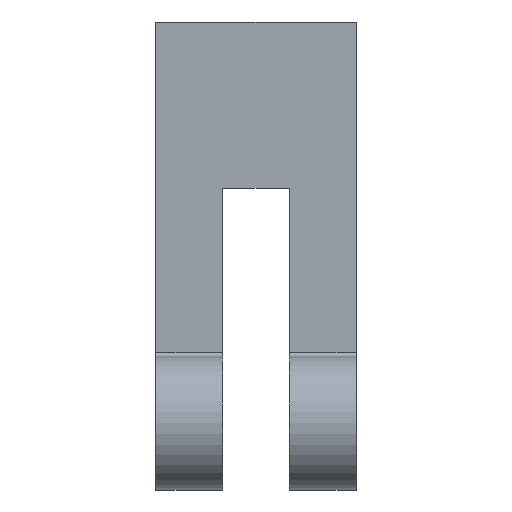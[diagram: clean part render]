
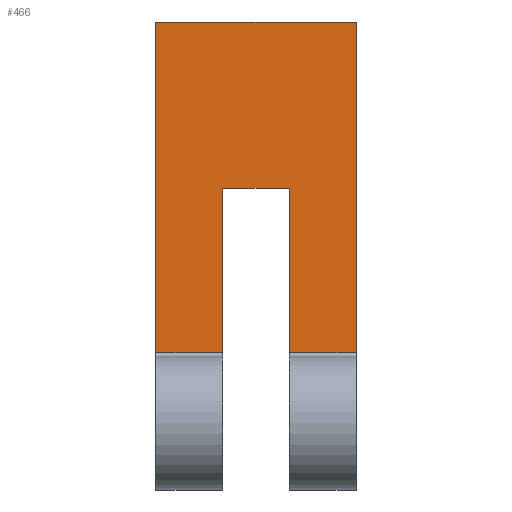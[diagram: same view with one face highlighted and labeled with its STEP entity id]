
A CAD part, top view. The second image highlights one B-rep face of the part: STEP entity #466.
In plain terms, the highlighted planar face has unit normal (0, 0, 1).
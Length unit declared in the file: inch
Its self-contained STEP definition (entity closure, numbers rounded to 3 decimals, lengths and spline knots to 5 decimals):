
#29=PLANE('',#520);
#52=FACE_OUTER_BOUND('',#76,.T.);
#76=EDGE_LOOP('',(#421,#422,#423,#424,#425,#426,#427,#428));
#80=LINE('',#664,#130);
#81=LINE('',#670,#131);
#91=LINE('',#705,#141);
#103=LINE('',#731,#153);
#124=LINE('',#778,#174);
#125=LINE('',#781,#175);
#127=LINE('',#784,#177);
#128=LINE('',#787,#178);
#130=VECTOR('',#532,0.3937);
#131=VECTOR('',#537,0.3937);
#141=VECTOR('',#567,0.3937);
#153=VECTOR('',#587,0.3937);
#174=VECTOR('',#638,0.3937);
#175=VECTOR('',#641,0.3937);
#177=VECTOR('',#645,0.3937);
#178=VECTOR('',#650,0.3937);
#195=VERTEX_POINT('',#657);
#198=VERTEX_POINT('',#662);
#200=VERTEX_POINT('',#667);
#201=VERTEX_POINT('',#669);
#216=VERTEX_POINT('',#704);
#226=VERTEX_POINT('',#730);
#237=VERTEX_POINT('',#776);
#238=VERTEX_POINT('',#780);
#242=EDGE_CURVE('',#195,#198,#80,.T.);
#244=EDGE_CURVE('',#201,#200,#81,.T.);
#261=EDGE_CURVE('',#216,#195,#91,.T.);
#275=EDGE_CURVE('',#201,#226,#103,.T.);
#299=EDGE_CURVE('',#237,#198,#124,.T.);
#300=EDGE_CURVE('',#238,#216,#125,.T.);
#302=EDGE_CURVE('',#200,#238,#127,.T.);
#304=EDGE_CURVE('',#226,#237,#128,.T.);
#421=ORIENTED_EDGE('',*,*,#242,.T.);
#422=ORIENTED_EDGE('',*,*,#299,.F.);
#423=ORIENTED_EDGE('',*,*,#304,.F.);
#424=ORIENTED_EDGE('',*,*,#275,.F.);
#425=ORIENTED_EDGE('',*,*,#244,.T.);
#426=ORIENTED_EDGE('',*,*,#302,.T.);
#427=ORIENTED_EDGE('',*,*,#300,.T.);
#428=ORIENTED_EDGE('',*,*,#261,.T.);
#466=ADVANCED_FACE('',(#52),#29,.F.);
#520=AXIS2_PLACEMENT_3D('',#786,#648,#649);
#532=DIRECTION('',(1.,0.,0.));
#537=DIRECTION('',(1.,0.,0.));
#567=DIRECTION('',(0.,-1.,0.));
#587=DIRECTION('',(0.,1.,0.));
#638=DIRECTION('',(0.,-1.,0.));
#641=DIRECTION('',(1.,0.,0.));
#645=DIRECTION('',(0.,1.,0.));
#648=DIRECTION('center_axis',(0.,0.,-1.));
#649=DIRECTION('ref_axis',(0.,-1.,0.));
#650=DIRECTION('',(1.,0.,0.));
#657=CARTESIAN_POINT('',(0.25,0.25644,0.1875));
#662=CARTESIAN_POINT('',(0.375,0.25644,0.1875));
#664=CARTESIAN_POINT('',(0.375,0.25644,0.1875));
#667=CARTESIAN_POINT('',(0.125,0.25644,0.1875));
#669=CARTESIAN_POINT('',(0.,0.25644,0.1875));
#670=CARTESIAN_POINT('',(0.375,0.25644,0.1875));
#704=CARTESIAN_POINT('',(0.25,0.56376,0.1875));
#705=CARTESIAN_POINT('',(0.25,0.71938,0.1875));
#730=CARTESIAN_POINT('',(0.,0.875,0.1875));
#731=CARTESIAN_POINT('',(0.,0.875,0.1875));
#776=CARTESIAN_POINT('',(0.375,0.875,0.1875));
#778=CARTESIAN_POINT('',(0.375,0.4375,0.1875));
#780=CARTESIAN_POINT('',(0.125,0.56376,0.1875));
#781=CARTESIAN_POINT('',(0.25,0.56376,0.1875));
#784=CARTESIAN_POINT('',(0.125,0.5625,0.1875));
#786=CARTESIAN_POINT('Origin',(0.375,0.875,0.1875));
#787=CARTESIAN_POINT('',(0.375,0.875,0.1875));
